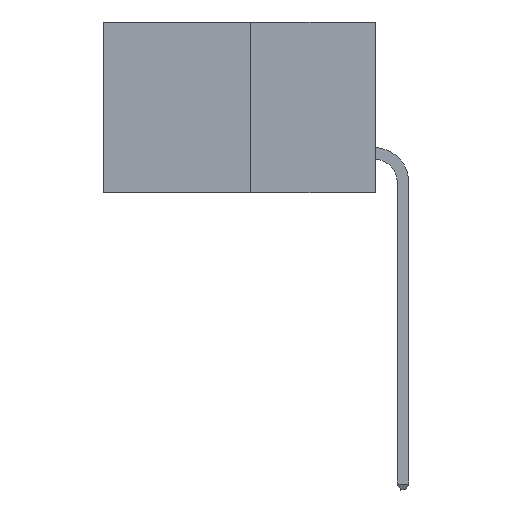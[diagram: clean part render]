
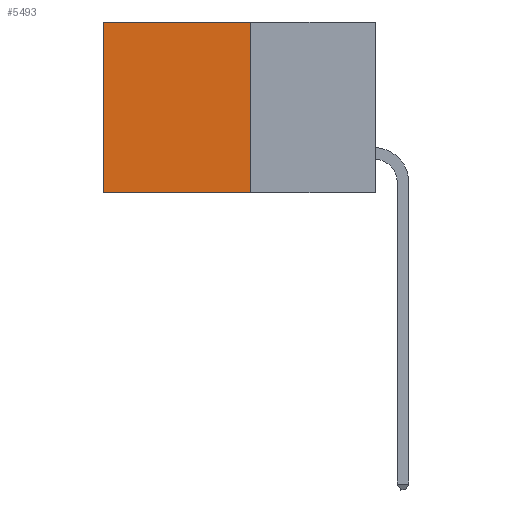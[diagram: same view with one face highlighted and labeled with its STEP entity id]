
A CAD part, left-side view. The second image highlights one B-rep face of the part: STEP entity #5493.
In plain terms, the highlighted planar face has unit normal (-1, 0, 0).
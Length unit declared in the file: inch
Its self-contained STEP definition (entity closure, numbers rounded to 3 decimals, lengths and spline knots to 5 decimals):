
#131 = EDGE_CURVE ( 'NONE', #7897, #4125, #4163, .T. ) ;
#481 = CARTESIAN_POINT ( 'NONE',  ( 0.277, 0.27, 0. ) ) ;
#677 = EDGE_CURVE ( 'NONE', #4125, #758, #6652, .T. ) ;
#713 = CARTESIAN_POINT ( 'NONE',  ( 0.277, 0.59, -0.37 ) ) ;
#731 = DIRECTION ( 'NONE',  ( 0., 0., -1. ) ) ;
#744 = DIRECTION ( 'NONE',  ( 1., 0., 0. ) ) ;
#758 = VERTEX_POINT ( 'NONE', #2971 ) ;
#778 = DIRECTION ( 'NONE',  ( 0., 0., -1. ) ) ;
#874 = PLANE ( 'NONE',  #4211 ) ;
#1220 = LINE ( 'NONE', #481, #12536 ) ;
#1787 = CARTESIAN_POINT ( 'NONE',  ( 0.277, 0.27, -0.37 ) ) ;
#1869 = VECTOR ( 'NONE', #4003, 39.37008 ) ;
#2352 = ORIENTED_EDGE ( 'NONE', *, *, #11594, .T. ) ;
#2354 = ORIENTED_EDGE ( 'NONE', *, *, #677, .F. ) ;
#2488 = ORIENTED_EDGE ( 'NONE', *, *, #131, .F. ) ;
#2511 = ORIENTED_EDGE ( 'NONE', *, *, #13214, .T. ) ;
#2971 = CARTESIAN_POINT ( 'NONE',  ( 0.277, 0.59, -0.37 ) ) ;
#3000 = VECTOR ( 'NONE', #6337, 39.37008 ) ;
#3385 = CARTESIAN_POINT ( 'NONE',  ( 0.277, 0.27, -0.37 ) ) ;
#4003 = DIRECTION ( 'NONE',  ( 0., 0., -1. ) ) ;
#4072 = EDGE_LOOP ( 'NONE', ( #2352, #2354, #2488, #2511 ) ) ;
#4125 = VERTEX_POINT ( 'NONE', #4572 ) ;
#4163 = LINE ( 'NONE', #3385, #12898 ) ;
#4211 = AXIS2_PLACEMENT_3D ( 'NONE', #1787, #744, #731 ) ;
#4572 = CARTESIAN_POINT ( 'NONE',  ( 0.277, 0.27, -0.37 ) ) ;
#4792 = LINE ( 'NONE', #713, #1869 ) ;
#5390 = CARTESIAN_POINT ( 'NONE',  ( 0.277, 0.27, -0.37 ) ) ;
#5493 = ADVANCED_FACE ( 'NONE', ( #11995 ), #874, .F. ) ;
#6337 = DIRECTION ( 'NONE',  ( 0., 1., 0. ) ) ;
#6652 = LINE ( 'NONE', #5390, #3000 ) ;
#6776 = VERTEX_POINT ( 'NONE', #12639 ) ;
#7100 = DIRECTION ( 'NONE',  ( 0., 1., 0. ) ) ;
#7897 = VERTEX_POINT ( 'NONE', #7998 ) ;
#7998 = CARTESIAN_POINT ( 'NONE',  ( 0.277, 0.27, 0. ) ) ;
#11594 = EDGE_CURVE ( 'NONE', #6776, #758, #4792, .T. ) ;
#11995 = FACE_OUTER_BOUND ( 'NONE', #4072, .T. ) ;
#12536 = VECTOR ( 'NONE', #7100, 39.37008 ) ;
#12639 = CARTESIAN_POINT ( 'NONE',  ( 0.277, 0.59, 0. ) ) ;
#12898 = VECTOR ( 'NONE', #778, 39.37008 ) ;
#13214 = EDGE_CURVE ( 'NONE', #7897, #6776, #1220, .T. ) ;
